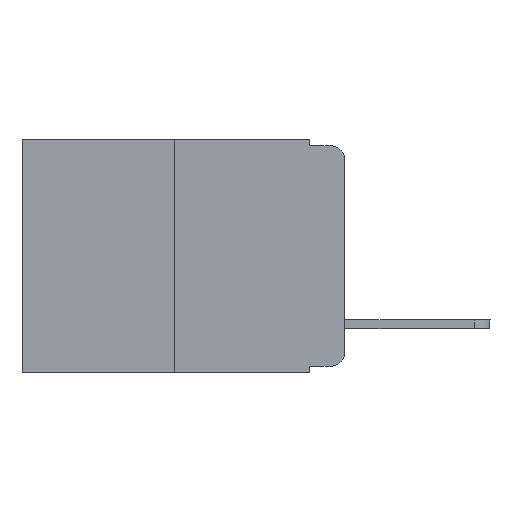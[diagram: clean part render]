
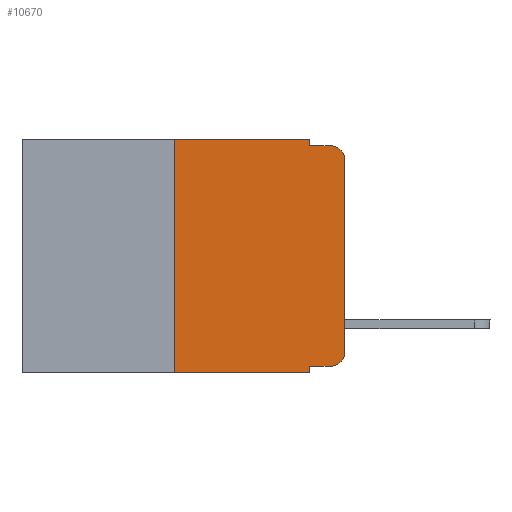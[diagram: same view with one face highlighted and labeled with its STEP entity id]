
A CAD part, left-side view. The second image highlights one B-rep face of the part: STEP entity #10670.
In plain terms, the highlighted planar face has unit normal (-1, 0, 0).
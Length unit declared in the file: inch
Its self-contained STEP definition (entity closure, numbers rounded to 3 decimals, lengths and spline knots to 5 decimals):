
#2 = CARTESIAN_POINT ( 'NONE',  ( 0., 0.02, -0.03 ) ) ;
#798 = EDGE_CURVE ( 'NONE', #1213, #8775, #14615, .T. ) ;
#1077 = DIRECTION ( 'NONE',  ( 0., 0., 1. ) ) ;
#1200 = VECTOR ( 'NONE', #13517, 39.37008 ) ;
#1213 = VERTEX_POINT ( 'NONE', #10449 ) ;
#1364 = CARTESIAN_POINT ( 'NONE',  ( 0., 0.051, -0.333 ) ) ;
#2001 = DIRECTION ( 'NONE',  ( 0., -1., 0. ) ) ;
#2099 = CARTESIAN_POINT ( 'NONE',  ( 0., 0.25, -0.343 ) ) ;
#2140 = DIRECTION ( 'NONE',  ( 0., -1., 0. ) ) ;
#2772 = EDGE_CURVE ( 'NONE', #3684, #4768, #9155, .T. ) ;
#3073 = CARTESIAN_POINT ( 'NONE',  ( 0., 0.473, 0. ) ) ;
#3094 = VERTEX_POINT ( 'NONE', #13503 ) ;
#3113 = ORIENTED_EDGE ( 'NONE', *, *, #10437, .F. ) ;
#3179 = VECTOR ( 'NONE', #8721, 39.37008 ) ;
#3237 = VERTEX_POINT ( 'NONE', #1364 ) ;
#3684 = VERTEX_POINT ( 'NONE', #4320 ) ;
#3784 = CARTESIAN_POINT ( 'NONE',  ( 0., 0.473, 0. ) ) ;
#3887 = EDGE_CURVE ( 'NONE', #3237, #14040, #13768, .T. ) ;
#4000 = CARTESIAN_POINT ( 'NONE',  ( 0., 0.02, -0.313 ) ) ;
#4187 = DIRECTION ( 'NONE',  ( -1., 0., 0. ) ) ;
#4320 = CARTESIAN_POINT ( 'NONE',  ( 0., 0.02, -0.333 ) ) ;
#4768 = VERTEX_POINT ( 'NONE', #15374 ) ;
#4911 = CARTESIAN_POINT ( 'NONE',  ( 0., 0.473, -0.343 ) ) ;
#5327 = DIRECTION ( 'NONE',  ( 0., 0., -1. ) ) ;
#5614 = LINE ( 'NONE', #4911, #1200 ) ;
#5688 = DIRECTION ( 'NONE',  ( 0., 0., -1. ) ) ;
#5737 = VECTOR ( 'NONE', #1077, 39.37008 ) ;
#5749 = DIRECTION ( 'NONE',  ( -1., 0., 0. ) ) ;
#6038 = EDGE_CURVE ( 'NONE', #3237, #3684, #10122, .T. ) ;
#6271 = VECTOR ( 'NONE', #14855, 39.37008 ) ;
#6906 = AXIS2_PLACEMENT_3D ( 'NONE', #4000, #4187, #13893 ) ;
#7284 = ORIENTED_EDGE ( 'NONE', *, *, #9095, .T. ) ;
#7354 = FACE_OUTER_BOUND ( 'NONE', #9960, .T. ) ;
#7526 = VECTOR ( 'NONE', #2140, 39.37008 ) ;
#7606 = AXIS2_PLACEMENT_3D ( 'NONE', #3073, #12776, #12973 ) ;
#7736 = LINE ( 'NONE', #11975, #5737 ) ;
#8234 = VERTEX_POINT ( 'NONE', #2099 ) ;
#8476 = EDGE_CURVE ( 'NONE', #8234, #15478, #14283, .T. ) ;
#8721 = DIRECTION ( 'NONE',  ( 0., 0., -1. ) ) ;
#8775 = VERTEX_POINT ( 'NONE', #10622 ) ;
#8801 = CARTESIAN_POINT ( 'NONE',  ( 0., 0.051, -0.333 ) ) ;
#9095 = EDGE_CURVE ( 'NONE', #8234, #14040, #5614, .T. ) ;
#9155 = CIRCLE ( 'NONE', #6906, 0.02 ) ;
#9196 = CARTESIAN_POINT ( 'NONE',  ( 0., 0.051, -0.01 ) ) ;
#9704 = ORIENTED_EDGE ( 'NONE', *, *, #2772, .T. ) ;
#9960 = EDGE_LOOP ( 'NONE', ( #17183, #16133, #12974, #15318, #3113, #13861, #7284, #12655, #12453, #9704 ) ) ;
#10090 = CARTESIAN_POINT ( 'NONE',  ( 0., 0.051, -0.343 ) ) ;
#10122 = LINE ( 'NONE', #8801, #12148 ) ;
#10159 = EDGE_CURVE ( 'NONE', #12191, #1213, #13380, .T. ) ;
#10437 = EDGE_CURVE ( 'NONE', #15478, #12191, #13817, .T. ) ;
#10449 = CARTESIAN_POINT ( 'NONE',  ( 0., 0.051, -0.01 ) ) ;
#10622 = CARTESIAN_POINT ( 'NONE',  ( 0., 0.02, -0.01 ) ) ;
#10670 = ADVANCED_FACE ( 'NONE', ( #7354 ), #13080, .F. ) ;
#10771 = CARTESIAN_POINT ( 'NONE',  ( 0., 0.051, 0. ) ) ;
#11691 = EDGE_CURVE ( 'NONE', #3094, #8775, #18184, .T. ) ;
#11975 = CARTESIAN_POINT ( 'NONE',  ( 0., 0., 0. ) ) ;
#12148 = VECTOR ( 'NONE', #2001, 39.37008 ) ;
#12191 = VERTEX_POINT ( 'NONE', #10771 ) ;
#12219 = VECTOR ( 'NONE', #5327, 39.37008 ) ;
#12312 = VECTOR ( 'NONE', #12556, 39.37008 ) ;
#12453 = ORIENTED_EDGE ( 'NONE', *, *, #6038, .T. ) ;
#12556 = DIRECTION ( 'NONE',  ( 0., 0., 1. ) ) ;
#12655 = ORIENTED_EDGE ( 'NONE', *, *, #3887, .F. ) ;
#12776 = DIRECTION ( 'NONE',  ( 1., 0., 0. ) ) ;
#12973 = DIRECTION ( 'NONE',  ( 0., 0., -1. ) ) ;
#12974 = ORIENTED_EDGE ( 'NONE', *, *, #798, .F. ) ;
#12996 = CARTESIAN_POINT ( 'NONE',  ( 0., 0.051, 0. ) ) ;
#13080 = PLANE ( 'NONE',  #7606 ) ;
#13380 = LINE ( 'NONE', #12996, #3179 ) ;
#13503 = CARTESIAN_POINT ( 'NONE',  ( 0., 0., -0.03 ) ) ;
#13517 = DIRECTION ( 'NONE',  ( 0., -1., 0. ) ) ;
#13768 = LINE ( 'NONE', #15171, #12219 ) ;
#13817 = LINE ( 'NONE', #3784, #6271 ) ;
#13861 = ORIENTED_EDGE ( 'NONE', *, *, #8476, .F. ) ;
#13893 = DIRECTION ( 'NONE',  ( 0., 0., -1. ) ) ;
#14040 = VERTEX_POINT ( 'NONE', #10090 ) ;
#14283 = LINE ( 'NONE', #16850, #12312 ) ;
#14615 = LINE ( 'NONE', #9196, #7526 ) ;
#14855 = DIRECTION ( 'NONE',  ( 0., -1., 0. ) ) ;
#15171 = CARTESIAN_POINT ( 'NONE',  ( 0., 0.051, 0. ) ) ;
#15318 = ORIENTED_EDGE ( 'NONE', *, *, #10159, .F. ) ;
#15374 = CARTESIAN_POINT ( 'NONE',  ( 0., 0., -0.313 ) ) ;
#15462 = AXIS2_PLACEMENT_3D ( 'NONE', #2, #5749, #5688 ) ;
#15478 = VERTEX_POINT ( 'NONE', #17733 ) ;
#16035 = EDGE_CURVE ( 'NONE', #4768, #3094, #7736, .T. ) ;
#16133 = ORIENTED_EDGE ( 'NONE', *, *, #11691, .T. ) ;
#16850 = CARTESIAN_POINT ( 'NONE',  ( 0., 0.25, 0. ) ) ;
#17183 = ORIENTED_EDGE ( 'NONE', *, *, #16035, .T. ) ;
#17733 = CARTESIAN_POINT ( 'NONE',  ( 0., 0.25, 0. ) ) ;
#18184 = CIRCLE ( 'NONE', #15462, 0.02 ) ;
